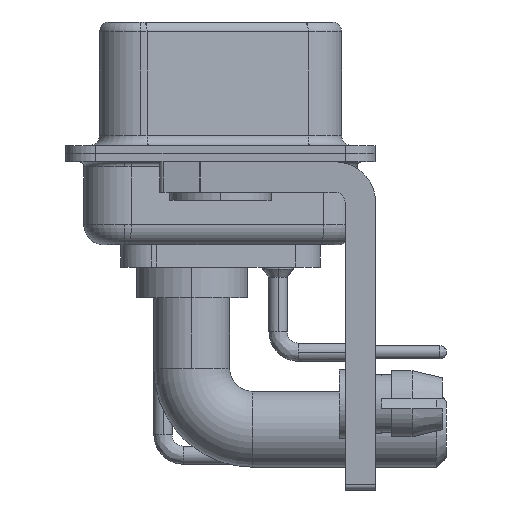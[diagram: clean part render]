
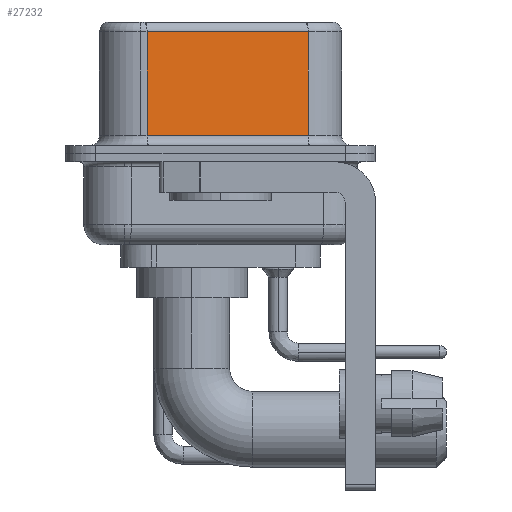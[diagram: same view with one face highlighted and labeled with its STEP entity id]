
A CAD part, left-side view. The second image highlights one B-rep face of the part: STEP entity #27232.
In plain terms, the highlighted planar face has unit normal (-0.985, -0.174, 0).
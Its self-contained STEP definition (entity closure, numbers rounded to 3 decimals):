
#2377 = EDGE_CURVE ( 'NONE', #20759, #12353, #12909, .T. ) ;
#2874 = DIRECTION ( 'NONE',  ( 0., 0., -1. ) ) ;
#3064 = CARTESIAN_POINT ( 'NONE',  ( 3.73, 3.628, 6.52 ) ) ;
#3562 = EDGE_CURVE ( 'NONE', #33774, #25905, #4441, .T. ) ;
#4441 = LINE ( 'NONE', #12777, #21816 ) ;
#4658 = DIRECTION ( 'NONE',  ( 0.985, 0.174, 0. ) ) ;
#6329 = ORIENTED_EDGE ( 'NONE', *, *, #34111, .F. ) ;
#6667 = CARTESIAN_POINT ( 'NONE',  ( 3.73, 3.628, 6.02 ) ) ;
#9616 = CARTESIAN_POINT ( 'NONE',  ( 5.132, -4.322, 6.52 ) ) ;
#10122 = DIRECTION ( 'NONE',  ( 0.174, -0.985, 0. ) ) ;
#12045 = EDGE_LOOP ( 'NONE', ( #6329, #24093, #20012, #31235 ) ) ;
#12353 = VERTEX_POINT ( 'NONE', #28108 ) ;
#12777 = CARTESIAN_POINT ( 'NONE',  ( 5.132, -4.322, 6.02 ) ) ;
#12909 = LINE ( 'NONE', #24043, #30536 ) ;
#13735 = CARTESIAN_POINT ( 'NONE',  ( 5.132, -4.322, 6.02 ) ) ;
#17206 = AXIS2_PLACEMENT_3D ( 'NONE', #32805, #4658, #29285 ) ;
#18151 = DIRECTION ( 'NONE',  ( 0., 0., -1. ) ) ;
#20012 = ORIENTED_EDGE ( 'NONE', *, *, #28292, .T. ) ;
#20566 = LINE ( 'NONE', #9616, #26191 ) ;
#20759 = VERTEX_POINT ( 'NONE', #35036 ) ;
#21511 = PLANE ( 'NONE',  #17206 ) ;
#21816 = VECTOR ( 'NONE', #35739, 1000. ) ;
#24043 = CARTESIAN_POINT ( 'NONE',  ( 5.132, -4.322, 0.9 ) ) ;
#24093 = ORIENTED_EDGE ( 'NONE', *, *, #3562, .T. ) ;
#25905 = VERTEX_POINT ( 'NONE', #6667 ) ;
#26191 = VECTOR ( 'NONE', #18151, 1000. ) ;
#26880 = FACE_OUTER_BOUND ( 'NONE', #12045, .T. ) ;
#27232 = ADVANCED_FACE ( 'NONE', ( #26880 ), #21511, .F. ) ;
#28108 = CARTESIAN_POINT ( 'NONE',  ( 5.132, -4.322, 0.9 ) ) ;
#28246 = LINE ( 'NONE', #3064, #34211 ) ;
#28292 = EDGE_CURVE ( 'NONE', #25905, #20759, #28246, .T. ) ;
#29285 = DIRECTION ( 'NONE',  ( -0.174, 0.985, 0. ) ) ;
#30536 = VECTOR ( 'NONE', #10122, 1000. ) ;
#31235 = ORIENTED_EDGE ( 'NONE', *, *, #2377, .T. ) ;
#32805 = CARTESIAN_POINT ( 'NONE',  ( 5.132, -4.322, 6.52 ) ) ;
#33774 = VERTEX_POINT ( 'NONE', #13735 ) ;
#34111 = EDGE_CURVE ( 'NONE', #33774, #12353, #20566, .T. ) ;
#34211 = VECTOR ( 'NONE', #2874, 1000. ) ;
#35036 = CARTESIAN_POINT ( 'NONE',  ( 3.73, 3.628, 0.9 ) ) ;
#35739 = DIRECTION ( 'NONE',  ( -0.174, 0.985, 0. ) ) ;
